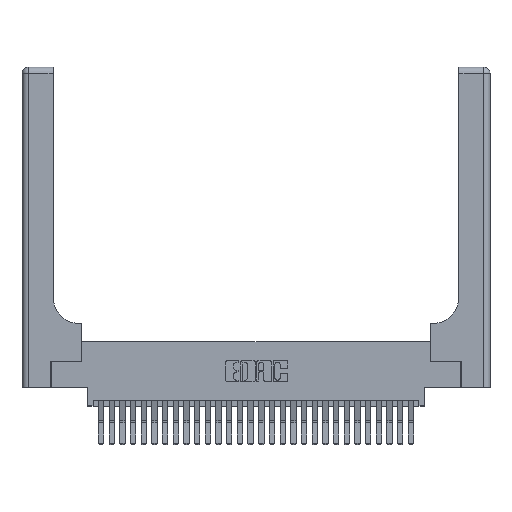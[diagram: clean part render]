
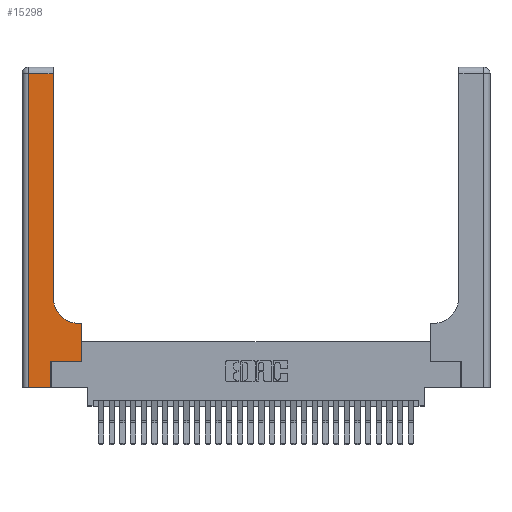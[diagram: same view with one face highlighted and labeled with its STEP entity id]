
A CAD part, top view. The second image highlights one B-rep face of the part: STEP entity #15298.
In plain terms, the highlighted planar face has unit normal (0, 0, 1).
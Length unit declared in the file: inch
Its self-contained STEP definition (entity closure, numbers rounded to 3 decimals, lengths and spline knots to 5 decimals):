
#66 = DIRECTION ( 'NONE',  ( -1., 0., 0. ) ) ;
#189 = EDGE_CURVE ( 'NONE', #26374, #18527, #8760, .T. ) ;
#675 = LINE ( 'NONE', #22269, #25964 ) ;
#1525 = VECTOR ( 'NONE', #4922, 39.37008 ) ;
#1763 = EDGE_CURVE ( 'NONE', #18527, #2281, #4079, .T. ) ;
#1824 = DIRECTION ( 'NONE',  ( 0., -1., 0. ) ) ;
#2043 = DIRECTION ( 'NONE',  ( 0., 0., -1. ) ) ;
#2281 = VERTEX_POINT ( 'NONE', #2820 ) ;
#2820 = CARTESIAN_POINT ( 'NONE',  ( 0.06, 2.94, 0.37 ) ) ;
#3827 = ORIENTED_EDGE ( 'NONE', *, *, #15532, .T. ) ;
#4079 = LINE ( 'NONE', #5822, #28450 ) ;
#4206 = EDGE_CURVE ( 'NONE', #14758, #10165, #4546, .T. ) ;
#4546 = LINE ( 'NONE', #12682, #21350 ) ;
#4922 = DIRECTION ( 'NONE',  ( 0., 1., 0. ) ) ;
#5070 = CARTESIAN_POINT ( 'NONE',  ( 0.269, 0., 0.37 ) ) ;
#5637 = EDGE_CURVE ( 'NONE', #2281, #14758, #21259, .T. ) ;
#5822 = CARTESIAN_POINT ( 'NONE',  ( 0., 2.94, 0.37 ) ) ;
#5950 = VECTOR ( 'NONE', #29203, 39.37008 ) ;
#6309 = CARTESIAN_POINT ( 'NONE',  ( 0.2915, 3., 0.37 ) ) ;
#8760 = LINE ( 'NONE', #6309, #1525 ) ;
#9400 = CARTESIAN_POINT ( 'NONE',  ( 0.06, 0., 0.37 ) ) ;
#10165 = VERTEX_POINT ( 'NONE', #5070 ) ;
#11209 = EDGE_CURVE ( 'NONE', #29860, #26374, #22570, .T. ) ;
#11851 = VERTEX_POINT ( 'NONE', #29972 ) ;
#12682 = CARTESIAN_POINT ( 'NONE',  ( 0., 0., 0.37 ) ) ;
#12941 = CARTESIAN_POINT ( 'NONE',  ( 0.269, 0., 0.37 ) ) ;
#13556 = ORIENTED_EDGE ( 'NONE', *, *, #189, .T. ) ;
#13663 = CARTESIAN_POINT ( 'NONE',  ( 0.2915, 2.94, 0.37 ) ) ;
#14261 = VECTOR ( 'NONE', #1824, 39.37008 ) ;
#14503 = DIRECTION ( 'NONE',  ( 0., 0., -1. ) ) ;
#14758 = VERTEX_POINT ( 'NONE', #9400 ) ;
#14804 = CARTESIAN_POINT ( 'NONE',  ( 0.5415, 0.6, 0.37 ) ) ;
#15088 = DIRECTION ( 'NONE',  ( 1., 0., 0. ) ) ;
#15204 = CARTESIAN_POINT ( 'NONE',  ( 0.5585, 0.6, 0.37 ) ) ;
#15298 = ADVANCED_FACE ( 'NONE', ( #19458 ), #28409, .F. ) ;
#15532 = EDGE_CURVE ( 'NONE', #19003, #29860, #675, .T. ) ;
#15608 = CARTESIAN_POINT ( 'NONE',  ( 0.2915, 0.85, 0.37 ) ) ;
#16245 = CARTESIAN_POINT ( 'NONE',  ( 0.06, 3., 0.37 ) ) ;
#16456 = CARTESIAN_POINT ( 'NONE',  ( 0.5415, 0.85, 0.37 ) ) ;
#16971 = DIRECTION ( 'NONE',  ( 0., 1., 0. ) ) ;
#17081 = ORIENTED_EDGE ( 'NONE', *, *, #23642, .T. ) ;
#17311 = ORIENTED_EDGE ( 'NONE', *, *, #5637, .T. ) ;
#17375 = CARTESIAN_POINT ( 'NONE',  ( 0.269, 0.25, 0.37 ) ) ;
#17569 = VECTOR ( 'NONE', #26612, 39.37008 ) ;
#18527 = VERTEX_POINT ( 'NONE', #13663 ) ;
#18812 = DIRECTION ( 'NONE',  ( 1., 0., 0. ) ) ;
#19003 = VERTEX_POINT ( 'NONE', #15204 ) ;
#19130 = CARTESIAN_POINT ( 'NONE',  ( 0., 3., 0.37 ) ) ;
#19349 = ORIENTED_EDGE ( 'NONE', *, *, #1763, .T. ) ;
#19458 = FACE_OUTER_BOUND ( 'NONE', #29428, .T. ) ;
#19734 = ORIENTED_EDGE ( 'NONE', *, *, #23681, .T. ) ;
#20337 = ORIENTED_EDGE ( 'NONE', *, *, #4206, .T. ) ;
#21102 = VECTOR ( 'NONE', #16971, 39.37008 ) ;
#21259 = LINE ( 'NONE', #16245, #14261 ) ;
#21350 = VECTOR ( 'NONE', #15088, 39.37008 ) ;
#21819 = LINE ( 'NONE', #28503, #21102 ) ;
#22167 = DIRECTION ( 'NONE',  ( -1., 0., 0. ) ) ;
#22269 = CARTESIAN_POINT ( 'NONE',  ( 0.2915, 0.6, 0.37 ) ) ;
#22570 = CIRCLE ( 'NONE', #24165, 0.25 ) ;
#23642 = EDGE_CURVE ( 'NONE', #11851, #29633, #29861, .T. ) ;
#23681 = EDGE_CURVE ( 'NONE', #10165, #11851, #24128, .T. ) ;
#24128 = LINE ( 'NONE', #12941, #5950 ) ;
#24165 = AXIS2_PLACEMENT_3D ( 'NONE', #16456, #2043, #18812 ) ;
#25004 = CARTESIAN_POINT ( 'NONE',  ( 0.5585, 0.25, 0.37 ) ) ;
#25964 = VECTOR ( 'NONE', #22167, 39.37008 ) ;
#26003 = ORIENTED_EDGE ( 'NONE', *, *, #11209, .T. ) ;
#26060 = EDGE_CURVE ( 'NONE', #29633, #19003, #21819, .T. ) ;
#26374 = VERTEX_POINT ( 'NONE', #15608 ) ;
#26612 = DIRECTION ( 'NONE',  ( 1., 0., 0. ) ) ;
#28066 = AXIS2_PLACEMENT_3D ( 'NONE', #19130, #14503, #66 ) ;
#28108 = ORIENTED_EDGE ( 'NONE', *, *, #26060, .T. ) ;
#28409 = PLANE ( 'NONE',  #28066 ) ;
#28450 = VECTOR ( 'NONE', #29372, 39.37008 ) ;
#28503 = CARTESIAN_POINT ( 'NONE',  ( 0.5585, 0.25, 0.37 ) ) ;
#29203 = DIRECTION ( 'NONE',  ( 0., 1., 0. ) ) ;
#29372 = DIRECTION ( 'NONE',  ( -1., 0., 0. ) ) ;
#29428 = EDGE_LOOP ( 'NONE', ( #13556, #19349, #17311, #20337, #19734, #17081, #28108, #3827, #26003 ) ) ;
#29633 = VERTEX_POINT ( 'NONE', #25004 ) ;
#29860 = VERTEX_POINT ( 'NONE', #14804 ) ;
#29861 = LINE ( 'NONE', #17375, #17569 ) ;
#29972 = CARTESIAN_POINT ( 'NONE',  ( 0.269, 0.25, 0.37 ) ) ;
